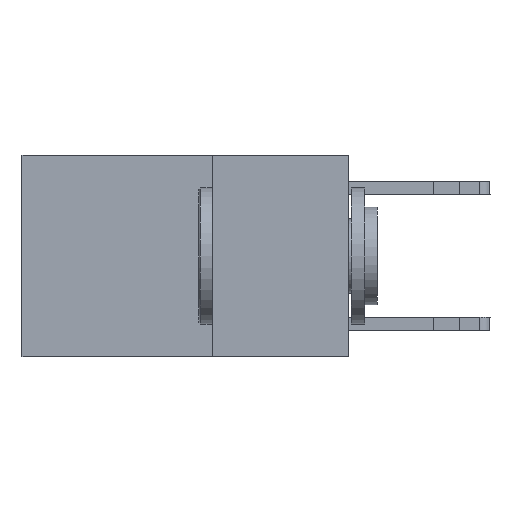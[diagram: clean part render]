
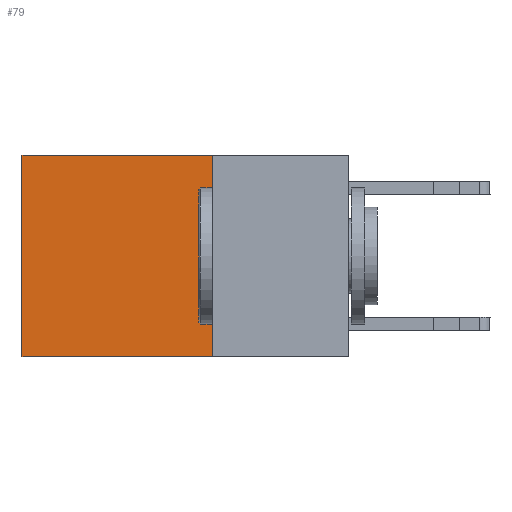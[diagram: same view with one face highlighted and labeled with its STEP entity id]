
A CAD part, left-side view. The second image highlights one B-rep face of the part: STEP entity #79.
In plain terms, the highlighted planar face has unit normal (-1, 0, 0).
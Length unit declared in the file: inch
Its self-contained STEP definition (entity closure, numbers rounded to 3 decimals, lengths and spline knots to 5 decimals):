
#79 = ADVANCED_FACE ( 'NONE', ( #13054 ), #507, .F. ) ;
#507 = PLANE ( 'NONE',  #8016 ) ;
#835 = VERTEX_POINT ( 'NONE', #8584 ) ;
#1222 = VERTEX_POINT ( 'NONE', #2422 ) ;
#1870 = CARTESIAN_POINT ( 'NONE',  ( 0.2625, 0.25, 0. ) ) ;
#2372 = ORIENTED_EDGE ( 'NONE', *, *, #9141, .T. ) ;
#2422 = CARTESIAN_POINT ( 'NONE',  ( 0.2625, 0.25, 0. ) ) ;
#2449 = CARTESIAN_POINT ( 'NONE',  ( 0.2625, 0.25, 0. ) ) ;
#3207 = DIRECTION ( 'NONE',  ( 0., 1., 0. ) ) ;
#3524 = VECTOR ( 'NONE', #3207, 39.37008 ) ;
#3964 = VERTEX_POINT ( 'NONE', #11633 ) ;
#4422 = CARTESIAN_POINT ( 'NONE',  ( 0.2625, 0.25, 0. ) ) ;
#4528 = LINE ( 'NONE', #2449, #12515 ) ;
#4738 = DIRECTION ( 'NONE',  ( 0., 1., 0. ) ) ;
#4971 = LINE ( 'NONE', #6817, #7497 ) ;
#5294 = LINE ( 'NONE', #8543, #3524 ) ;
#5551 = EDGE_CURVE ( 'NONE', #1222, #3964, #11684, .T. ) ;
#5836 = ORIENTED_EDGE ( 'NONE', *, *, #5551, .F. ) ;
#5952 = EDGE_CURVE ( 'NONE', #3964, #10941, #5294, .T. ) ;
#6453 = EDGE_LOOP ( 'NONE', ( #2372, #10959, #5836, #9107 ) ) ;
#6817 = CARTESIAN_POINT ( 'NONE',  ( 0.2625, 0.6, 0. ) ) ;
#7497 = VECTOR ( 'NONE', #10056, 39.37008 ) ;
#7832 = DIRECTION ( 'NONE',  ( 0., 0., -1. ) ) ;
#8016 = AXIS2_PLACEMENT_3D ( 'NONE', #1870, #8763, #7832 ) ;
#8543 = CARTESIAN_POINT ( 'NONE',  ( 0.2625, 0.25, -0.37 ) ) ;
#8558 = DIRECTION ( 'NONE',  ( 0., 0., -1. ) ) ;
#8584 = CARTESIAN_POINT ( 'NONE',  ( 0.2625, 0.6, 0. ) ) ;
#8763 = DIRECTION ( 'NONE',  ( 1., 0., 0. ) ) ;
#9107 = ORIENTED_EDGE ( 'NONE', *, *, #13010, .T. ) ;
#9141 = EDGE_CURVE ( 'NONE', #835, #10941, #4971, .T. ) ;
#10056 = DIRECTION ( 'NONE',  ( 0., 0., -1. ) ) ;
#10680 = VECTOR ( 'NONE', #8558, 39.37008 ) ;
#10941 = VERTEX_POINT ( 'NONE', #12011 ) ;
#10959 = ORIENTED_EDGE ( 'NONE', *, *, #5952, .F. ) ;
#11633 = CARTESIAN_POINT ( 'NONE',  ( 0.2625, 0.25, -0.37 ) ) ;
#11684 = LINE ( 'NONE', #4422, #10680 ) ;
#12011 = CARTESIAN_POINT ( 'NONE',  ( 0.2625, 0.6, -0.37 ) ) ;
#12515 = VECTOR ( 'NONE', #4738, 39.37008 ) ;
#13010 = EDGE_CURVE ( 'NONE', #1222, #835, #4528, .T. ) ;
#13054 = FACE_OUTER_BOUND ( 'NONE', #6453, .T. ) ;
